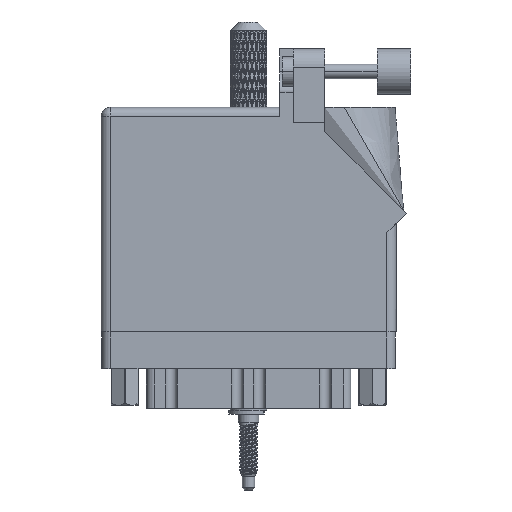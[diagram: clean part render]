
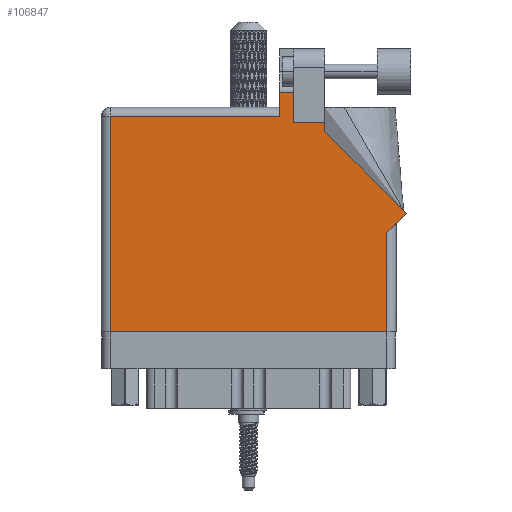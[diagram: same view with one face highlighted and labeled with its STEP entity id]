
A CAD part, front view. The second image highlights one B-rep face of the part: STEP entity #106847.
In plain terms, the highlighted face is planar.
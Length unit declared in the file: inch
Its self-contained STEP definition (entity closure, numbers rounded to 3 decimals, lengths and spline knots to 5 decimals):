
#197 = ORIENTED_EDGE ( 'NONE', *, *, #99733, .T. ) ;
#1721 = VERTEX_POINT ( 'NONE', #45065 ) ;
#2308 = LINE ( 'NONE', #38445, #28206 ) ;
#2905 = CARTESIAN_POINT ( 'NONE',  ( 1.524, 1.43, 0. ) ) ;
#4617 = VECTOR ( 'NONE', #94453, 39.37008 ) ;
#8092 = CARTESIAN_POINT ( 'NONE',  ( 2.08071, 0.80771, 0. ) ) ;
#8800 = ORIENTED_EDGE ( 'NONE', *, *, #112304, .T. ) ;
#9104 = VERTEX_POINT ( 'NONE', #99007 ) ;
#10945 = EDGE_CURVE ( 'NONE', #1721, #54573, #2308, .T. ) ;
#11406 = CARTESIAN_POINT ( 'NONE',  ( 0., 1.468, 0. ) ) ;
#12702 = ORIENTED_EDGE ( 'NONE', *, *, #107319, .T. ) ;
#13150 = VERTEX_POINT ( 'NONE', #15862 ) ;
#15862 = CARTESIAN_POINT ( 'NONE',  ( 1.311, 1.6315, 0. ) ) ;
#15954 = EDGE_CURVE ( 'NONE', #56925, #89454, #27472, .T. ) ;
#17132 = ORIENTED_EDGE ( 'NONE', *, *, #10945, .T. ) ;
#23326 = VECTOR ( 'NONE', #107260, 39.37008 ) ;
#24236 = CARTESIAN_POINT ( 'NONE',  ( 0.062, 0., 0. ) ) ;
#25289 = DIRECTION ( 'NONE',  ( 0., 1., 0. ) ) ;
#25461 = ORIENTED_EDGE ( 'NONE', *, *, #105606, .T. ) ;
#25890 = ORIENTED_EDGE ( 'NONE', *, *, #110568, .T. ) ;
#26578 = VERTEX_POINT ( 'NONE', #57769 ) ;
#27109 = CARTESIAN_POINT ( 'NONE',  ( 1.948, 0.737, 0. ) ) ;
#27472 = LINE ( 'NONE', #97490, #23326 ) ;
#28206 = VECTOR ( 'NONE', #37326, 39.37008 ) ;
#29138 = CARTESIAN_POINT ( 'NONE',  ( 1.524, 1.43, 0. ) ) ;
#33459 = DIRECTION ( 'NONE',  ( -0.707, 0.707, 0. ) ) ;
#34605 = LINE ( 'NONE', #27109, #56745 ) ;
#35359 = ORIENTED_EDGE ( 'NONE', *, *, #82366, .T. ) ;
#36456 = VECTOR ( 'NONE', #42322, 39.37008 ) ;
#36739 = CARTESIAN_POINT ( 'NONE',  ( 1.64177, 1.6315, 0. ) ) ;
#37104 = VERTEX_POINT ( 'NONE', #72189 ) ;
#37326 = DIRECTION ( 'NONE',  ( 0.707, 0.707, 0. ) ) ;
#37738 = AXIS2_PLACEMENT_3D ( 'NONE', #90910, #38687, #89764 ) ;
#38445 = CARTESIAN_POINT ( 'NONE',  ( 2.01, 0.737, 0. ) ) ;
#38687 = DIRECTION ( 'NONE',  ( 0., 0., -1. ) ) ;
#41382 = VECTOR ( 'NONE', #57196, 39.37008 ) ;
#41511 = DIRECTION ( 'NONE',  ( 0., -1., 0. ) ) ;
#42322 = DIRECTION ( 'NONE',  ( 1., 0., 0. ) ) ;
#45065 = CARTESIAN_POINT ( 'NONE',  ( 1.948, 0.675, 0. ) ) ;
#46434 = DIRECTION ( 'NONE',  ( -1., 0., 0. ) ) ;
#47226 = EDGE_CURVE ( 'NONE', #54573, #26578, #77050, .T. ) ;
#47499 = DIRECTION ( 'NONE',  ( -1., 0., 0. ) ) ;
#48125 = LINE ( 'NONE', #11406, #94143 ) ;
#50357 = LINE ( 'NONE', #68667, #36456 ) ;
#53809 = EDGE_CURVE ( 'NONE', #89454, #9104, #48125, .T. ) ;
#54573 = VERTEX_POINT ( 'NONE', #8092 ) ;
#55254 = ORIENTED_EDGE ( 'NONE', *, *, #53809, .T. ) ;
#55894 = PLANE ( 'NONE',  #37738 ) ;
#56745 = VECTOR ( 'NONE', #104655, 39.37008 ) ;
#56925 = VERTEX_POINT ( 'NONE', #106739 ) ;
#57196 = DIRECTION ( 'NONE',  ( -1., 0., 0. ) ) ;
#57769 = CARTESIAN_POINT ( 'NONE',  ( 1.524, 1.36442, 0. ) ) ;
#58228 = VERTEX_POINT ( 'NONE', #105179 ) ;
#60708 = CARTESIAN_POINT ( 'NONE',  ( 0.062, 0., 0. ) ) ;
#61966 = LINE ( 'NONE', #96994, #112460 ) ;
#68667 = CARTESIAN_POINT ( 'NONE',  ( 0., 0., 0. ) ) ;
#70116 = CARTESIAN_POINT ( 'NONE',  ( 2.08071, 0.80771, 0. ) ) ;
#70657 = VECTOR ( 'NONE', #47499, 39.37008 ) ;
#71148 = LINE ( 'NONE', #36739, #41382 ) ;
#71714 = VERTEX_POINT ( 'NONE', #2905 ) ;
#71965 = FACE_OUTER_BOUND ( 'NONE', #77633, .T. ) ;
#72189 = CARTESIAN_POINT ( 'NONE',  ( 1.948, 0., 0. ) ) ;
#77050 = LINE ( 'NONE', #70116, #104165 ) ;
#77633 = EDGE_LOOP ( 'NONE', ( #25461, #197, #78142, #55254, #25890, #35359, #110613, #17132, #81695, #8800, #12702 ) ) ;
#78142 = ORIENTED_EDGE ( 'NONE', *, *, #15954, .T. ) ;
#80816 = LINE ( 'NONE', #29138, #70657 ) ;
#81695 = ORIENTED_EDGE ( 'NONE', *, *, #47226, .T. ) ;
#82366 = EDGE_CURVE ( 'NONE', #85049, #37104, #50357, .T. ) ;
#85049 = VERTEX_POINT ( 'NONE', #60708 ) ;
#85554 = EDGE_CURVE ( 'NONE', #37104, #1721, #34605, .T. ) ;
#89454 = VERTEX_POINT ( 'NONE', #113051 ) ;
#89764 = DIRECTION ( 'NONE',  ( -1., 0., 0. ) ) ;
#90910 = CARTESIAN_POINT ( 'NONE',  ( 0., 1.53, 0. ) ) ;
#93134 = LINE ( 'NONE', #24236, #109190 ) ;
#94143 = VECTOR ( 'NONE', #46434, 39.37008 ) ;
#94453 = DIRECTION ( 'NONE',  ( 0., 1., 0. ) ) ;
#96994 = CARTESIAN_POINT ( 'NONE',  ( 1.524, 1.36442, 0. ) ) ;
#97490 = CARTESIAN_POINT ( 'NONE',  ( 1.217, 1.53, 0. ) ) ;
#99007 = CARTESIAN_POINT ( 'NONE',  ( 0.062, 1.468, 0. ) ) ;
#99733 = EDGE_CURVE ( 'NONE', #13150, #56925, #71148, .T. ) ;
#101352 = CARTESIAN_POINT ( 'NONE',  ( 1.311, 1.43, 0. ) ) ;
#104165 = VECTOR ( 'NONE', #33459, 39.37008 ) ;
#104655 = DIRECTION ( 'NONE',  ( 0., 1., 0. ) ) ;
#105179 = CARTESIAN_POINT ( 'NONE',  ( 1.311, 1.43, 0. ) ) ;
#105606 = EDGE_CURVE ( 'NONE', #58228, #13150, #110579, .T. ) ;
#106739 = CARTESIAN_POINT ( 'NONE',  ( 1.217, 1.6315, 0. ) ) ;
#106847 = ADVANCED_FACE ( 'NONE', ( #71965 ), #55894, .F. ) ;
#107260 = DIRECTION ( 'NONE',  ( 0., -1., 0. ) ) ;
#107319 = EDGE_CURVE ( 'NONE', #71714, #58228, #80816, .T. ) ;
#109190 = VECTOR ( 'NONE', #41511, 39.37008 ) ;
#110568 = EDGE_CURVE ( 'NONE', #9104, #85049, #93134, .T. ) ;
#110579 = LINE ( 'NONE', #101352, #4617 ) ;
#110613 = ORIENTED_EDGE ( 'NONE', *, *, #85554, .T. ) ;
#112304 = EDGE_CURVE ( 'NONE', #26578, #71714, #61966, .T. ) ;
#112460 = VECTOR ( 'NONE', #25289, 39.37008 ) ;
#113051 = CARTESIAN_POINT ( 'NONE',  ( 1.217, 1.468, 0. ) ) ;
